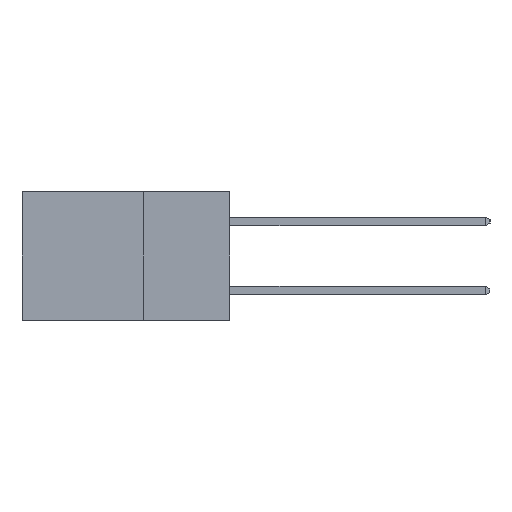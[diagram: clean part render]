
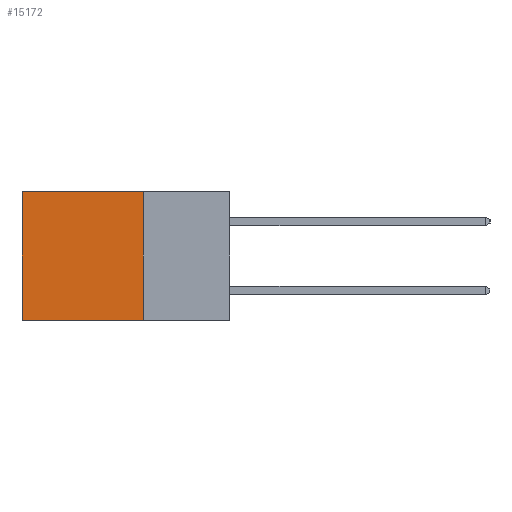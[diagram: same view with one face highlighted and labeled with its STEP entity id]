
A CAD part, left-side view. The second image highlights one B-rep face of the part: STEP entity #15172.
In plain terms, the highlighted planar face has unit normal (-1, 0, 0).
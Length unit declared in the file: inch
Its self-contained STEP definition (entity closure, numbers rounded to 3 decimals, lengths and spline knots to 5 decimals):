
#2308 = FACE_OUTER_BOUND ( 'NONE', #10000, .T. ) ;
#6601 = LINE ( 'NONE', #18244, #12031 ) ;
#7507 = ORIENTED_EDGE ( 'NONE', *, *, #22286, .T. ) ;
#9436 = VECTOR ( 'NONE', #28258, 39.37008 ) ;
#9988 = VERTEX_POINT ( 'NONE', #16595 ) ;
#10000 = EDGE_LOOP ( 'NONE', ( #7507, #18096, #26348, #13356 ) ) ;
#11168 = AXIS2_PLACEMENT_3D ( 'NONE', #13772, #25276, #11583 ) ;
#11193 = CARTESIAN_POINT ( 'NONE',  ( 0.298, 0.25, -0.37 ) ) ;
#11583 = DIRECTION ( 'NONE',  ( 0., 0., -1. ) ) ;
#12031 = VECTOR ( 'NONE', #22961, 39.37008 ) ;
#13356 = ORIENTED_EDGE ( 'NONE', *, *, #14235, .T. ) ;
#13772 = CARTESIAN_POINT ( 'NONE',  ( 0.298, 0.25, 0. ) ) ;
#13961 = VECTOR ( 'NONE', #28962, 39.37008 ) ;
#14235 = EDGE_CURVE ( 'NONE', #23071, #28647, #26114, .T. ) ;
#15076 = CARTESIAN_POINT ( 'NONE',  ( 0.298, 0.6, 0. ) ) ;
#15172 = ADVANCED_FACE ( 'NONE', ( #2308 ), #23017, .F. ) ;
#15357 = CARTESIAN_POINT ( 'NONE',  ( 0.298, 0.25, 0. ) ) ;
#16595 = CARTESIAN_POINT ( 'NONE',  ( 0.298, 0.25, -0.37 ) ) ;
#16978 = EDGE_CURVE ( 'NONE', #9988, #21423, #17744, .T. ) ;
#17744 = LINE ( 'NONE', #11193, #24544 ) ;
#18096 = ORIENTED_EDGE ( 'NONE', *, *, #16978, .F. ) ;
#18244 = CARTESIAN_POINT ( 'NONE',  ( 0.298, 0.6, 0. ) ) ;
#19213 = CARTESIAN_POINT ( 'NONE',  ( 0.298, 0.25, 0. ) ) ;
#20086 = CARTESIAN_POINT ( 'NONE',  ( 0.298, 0.6, -0.37 ) ) ;
#20898 = CARTESIAN_POINT ( 'NONE',  ( 0.298, 0.25, 0. ) ) ;
#21423 = VERTEX_POINT ( 'NONE', #20086 ) ;
#22286 = EDGE_CURVE ( 'NONE', #28647, #21423, #6601, .T. ) ;
#22961 = DIRECTION ( 'NONE',  ( 0., 0., -1. ) ) ;
#23017 = PLANE ( 'NONE',  #11168 ) ;
#23071 = VERTEX_POINT ( 'NONE', #20898 ) ;
#24544 = VECTOR ( 'NONE', #29307, 39.37008 ) ;
#24637 = EDGE_CURVE ( 'NONE', #23071, #9988, #28351, .T. ) ;
#25276 = DIRECTION ( 'NONE',  ( 1., 0., 0. ) ) ;
#26114 = LINE ( 'NONE', #15357, #13961 ) ;
#26348 = ORIENTED_EDGE ( 'NONE', *, *, #24637, .F. ) ;
#28258 = DIRECTION ( 'NONE',  ( 0., 0., -1. ) ) ;
#28351 = LINE ( 'NONE', #19213, #9436 ) ;
#28647 = VERTEX_POINT ( 'NONE', #15076 ) ;
#28962 = DIRECTION ( 'NONE',  ( 0., 1., 0. ) ) ;
#29307 = DIRECTION ( 'NONE',  ( 0., 1., 0. ) ) ;
